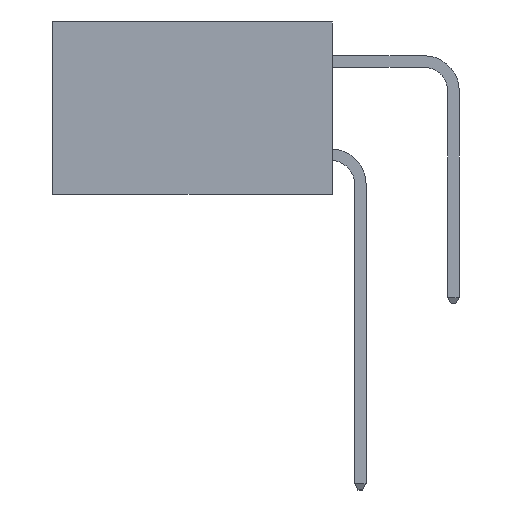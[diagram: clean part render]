
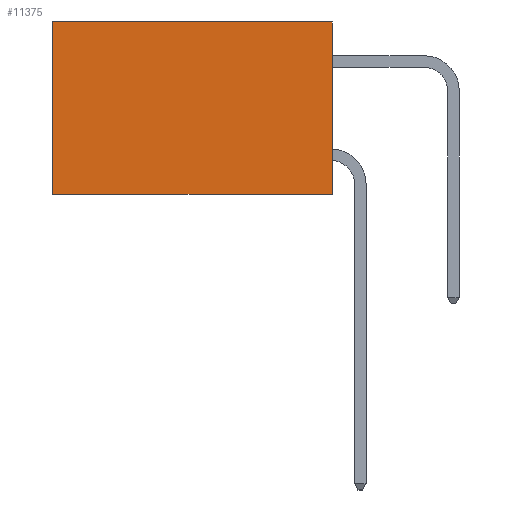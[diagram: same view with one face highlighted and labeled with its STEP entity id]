
A CAD part, left-side view. The second image highlights one B-rep face of the part: STEP entity #11375.
In plain terms, the highlighted planar face has unit normal (-1, 0, 0).
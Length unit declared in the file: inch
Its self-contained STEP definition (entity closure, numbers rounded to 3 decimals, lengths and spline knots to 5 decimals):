
#111 = VECTOR ( 'NONE', #11441, 39.37008 ) ;
#572 = EDGE_LOOP ( 'NONE', ( #12875, #7635, #2590, #5999 ) ) ;
#857 = EDGE_CURVE ( 'NONE', #12903, #14036, #4681, .T. ) ;
#2590 = ORIENTED_EDGE ( 'NONE', *, *, #13882, .F. ) ;
#3077 = CARTESIAN_POINT ( 'NONE',  ( 0.2615, 0.6, -0.37 ) ) ;
#4119 = VECTOR ( 'NONE', #11305, 39.37008 ) ;
#4227 = PLANE ( 'NONE',  #12002 ) ;
#4681 = LINE ( 'NONE', #9952, #10666 ) ;
#5603 = CARTESIAN_POINT ( 'NONE',  ( 0.2615, 0., 0. ) ) ;
#5701 = LINE ( 'NONE', #11952, #4119 ) ;
#5999 = ORIENTED_EDGE ( 'NONE', *, *, #11550, .T. ) ;
#6745 = CARTESIAN_POINT ( 'NONE',  ( 0.2615, 0., -0.37 ) ) ;
#6774 = CARTESIAN_POINT ( 'NONE',  ( 0.2615, 0., -0.37 ) ) ;
#7025 = DIRECTION ( 'NONE',  ( 1., 0., 0. ) ) ;
#7472 = DIRECTION ( 'NONE',  ( 0., 0., -1. ) ) ;
#7602 = VECTOR ( 'NONE', #7933, 39.37008 ) ;
#7635 = ORIENTED_EDGE ( 'NONE', *, *, #8722, .F. ) ;
#7933 = DIRECTION ( 'NONE',  ( 0., 0., -1. ) ) ;
#8722 = EDGE_CURVE ( 'NONE', #9846, #14036, #5701, .T. ) ;
#8894 = DIRECTION ( 'NONE',  ( 0., 0., -1. ) ) ;
#9522 = LINE ( 'NONE', #11876, #111 ) ;
#9846 = VERTEX_POINT ( 'NONE', #13644 ) ;
#9952 = CARTESIAN_POINT ( 'NONE',  ( 0.2615, 0.6, -0.37 ) ) ;
#10666 = VECTOR ( 'NONE', #8894, 39.37008 ) ;
#10702 = LINE ( 'NONE', #6745, #7602 ) ;
#11305 = DIRECTION ( 'NONE',  ( 0., 1., 0. ) ) ;
#11375 = ADVANCED_FACE ( 'NONE', ( #13971 ), #4227, .F. ) ;
#11441 = DIRECTION ( 'NONE',  ( 0., 1., 0. ) ) ;
#11550 = EDGE_CURVE ( 'NONE', #15537, #12903, #9522, .T. ) ;
#11876 = CARTESIAN_POINT ( 'NONE',  ( 0.2615, 0., 0. ) ) ;
#11952 = CARTESIAN_POINT ( 'NONE',  ( 0.2615, 0., -0.37 ) ) ;
#12002 = AXIS2_PLACEMENT_3D ( 'NONE', #6774, #7025, #7472 ) ;
#12112 = CARTESIAN_POINT ( 'NONE',  ( 0.2615, 0.6, 0. ) ) ;
#12875 = ORIENTED_EDGE ( 'NONE', *, *, #857, .T. ) ;
#12903 = VERTEX_POINT ( 'NONE', #12112 ) ;
#13644 = CARTESIAN_POINT ( 'NONE',  ( 0.2615, 0., -0.37 ) ) ;
#13882 = EDGE_CURVE ( 'NONE', #15537, #9846, #10702, .T. ) ;
#13971 = FACE_OUTER_BOUND ( 'NONE', #572, .T. ) ;
#14036 = VERTEX_POINT ( 'NONE', #3077 ) ;
#15537 = VERTEX_POINT ( 'NONE', #5603 ) ;
